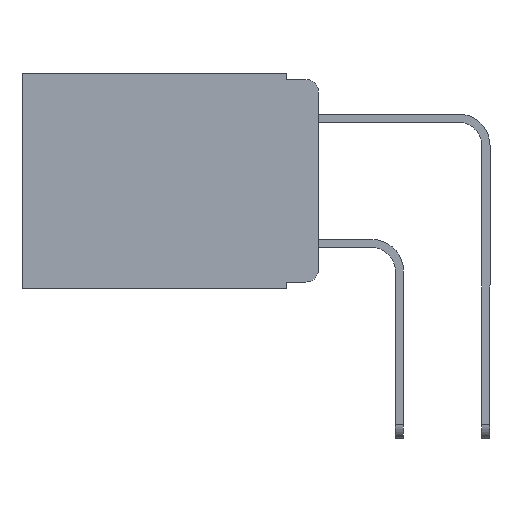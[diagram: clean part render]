
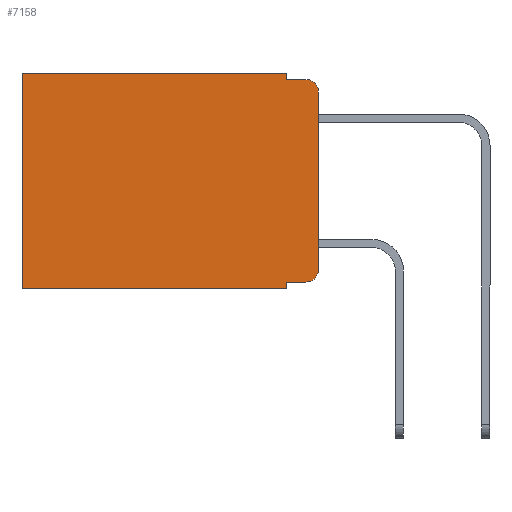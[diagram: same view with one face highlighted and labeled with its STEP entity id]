
A CAD part, left-side view. The second image highlights one B-rep face of the part: STEP entity #7158.
In plain terms, the highlighted planar face has unit normal (-1, 0, 0).
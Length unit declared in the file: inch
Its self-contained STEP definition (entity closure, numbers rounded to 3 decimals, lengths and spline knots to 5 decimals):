
#223 = ORIENTED_EDGE ( 'NONE', *, *, #5696, .T. ) ;
#335 = VERTEX_POINT ( 'NONE', #11684 ) ;
#1074 = VERTEX_POINT ( 'NONE', #4058 ) ;
#1845 = VERTEX_POINT ( 'NONE', #11970 ) ;
#2031 = CARTESIAN_POINT ( 'NONE',  ( 0.298, 0.051, -0.01 ) ) ;
#2078 = LINE ( 'NONE', #12561, #13362 ) ;
#2335 = CARTESIAN_POINT ( 'NONE',  ( 0.298, 0.051, 0. ) ) ;
#2446 = VECTOR ( 'NONE', #4903, 39.37008 ) ;
#2692 = DIRECTION ( 'NONE',  ( 0., 1., 0. ) ) ;
#2840 = LINE ( 'NONE', #9837, #10707 ) ;
#3233 = LINE ( 'NONE', #10443, #6314 ) ;
#3325 = PLANE ( 'NONE',  #10552 ) ;
#3360 = EDGE_CURVE ( 'NONE', #9661, #1074, #3486, .T. ) ;
#3486 = CIRCLE ( 'NONE', #14218, 0.02 ) ;
#3737 = CARTESIAN_POINT ( 'NONE',  ( 0.298, 0.051, -0.01 ) ) ;
#4058 = CARTESIAN_POINT ( 'NONE',  ( 0.298, 0., -0.313 ) ) ;
#4178 = EDGE_CURVE ( 'NONE', #1845, #9661, #5312, .T. ) ;
#4342 = DIRECTION ( 'NONE',  ( 0., 1., 0. ) ) ;
#4356 = VERTEX_POINT ( 'NONE', #3737 ) ;
#4550 = DIRECTION ( 'NONE',  ( 1., 0., 0. ) ) ;
#4607 = VERTEX_POINT ( 'NONE', #6567 ) ;
#4618 = CARTESIAN_POINT ( 'NONE',  ( 0.298, 0.473, 0. ) ) ;
#4702 = VECTOR ( 'NONE', #11023, 39.37008 ) ;
#4903 = DIRECTION ( 'NONE',  ( 0., 0., -1. ) ) ;
#4949 = VECTOR ( 'NONE', #11162, 39.37008 ) ;
#4968 = EDGE_CURVE ( 'NONE', #1845, #9438, #3233, .T. ) ;
#4982 = ORIENTED_EDGE ( 'NONE', *, *, #7124, .F. ) ;
#5066 = EDGE_CURVE ( 'NONE', #7900, #9487, #2078, .T. ) ;
#5312 = LINE ( 'NONE', #10072, #4949 ) ;
#5460 = CARTESIAN_POINT ( 'NONE',  ( 0.298, 0.02, -0.313 ) ) ;
#5696 = EDGE_CURVE ( 'NONE', #9487, #12836, #7772, .T. ) ;
#5735 = DIRECTION ( 'NONE',  ( -1., 0., 0. ) ) ;
#5866 = CARTESIAN_POINT ( 'NONE',  ( 0.298, 0.051, 0. ) ) ;
#5968 = LINE ( 'NONE', #10895, #12598 ) ;
#6314 = VECTOR ( 'NONE', #13435, 39.37008 ) ;
#6437 = EDGE_CURVE ( 'NONE', #7900, #4356, #7913, .T. ) ;
#6533 = ORIENTED_EDGE ( 'NONE', *, *, #6437, .F. ) ;
#6555 = DIRECTION ( 'NONE',  ( 0., 0., -1. ) ) ;
#6567 = CARTESIAN_POINT ( 'NONE',  ( 0.298, 0.02, -0.01 ) ) ;
#7124 = EDGE_CURVE ( 'NONE', #4356, #4607, #7585, .T. ) ;
#7158 = ADVANCED_FACE ( 'NONE', ( #7235 ), #3325, .F. ) ;
#7235 = FACE_OUTER_BOUND ( 'NONE', #9137, .T. ) ;
#7581 = VECTOR ( 'NONE', #14245, 39.37008 ) ;
#7585 = LINE ( 'NONE', #2031, #4702 ) ;
#7772 = LINE ( 'NONE', #10321, #2446 ) ;
#7847 = EDGE_CURVE ( 'NONE', #335, #4607, #8940, .T. ) ;
#7900 = VERTEX_POINT ( 'NONE', #2335 ) ;
#7913 = LINE ( 'NONE', #5866, #7581 ) ;
#8059 = CARTESIAN_POINT ( 'NONE',  ( 0.298, 0.02, -0.333 ) ) ;
#8377 = ORIENTED_EDGE ( 'NONE', *, *, #12076, .F. ) ;
#8737 = ORIENTED_EDGE ( 'NONE', *, *, #12150, .F. ) ;
#8831 = CARTESIAN_POINT ( 'NONE',  ( 0.298, 0.473, -0.343 ) ) ;
#8940 = CIRCLE ( 'NONE', #10730, 0.02 ) ;
#9137 = EDGE_LOOP ( 'NONE', ( #8737, #13190, #4982, #6533, #12044, #223, #8377, #13023, #14110, #10239 ) ) ;
#9438 = VERTEX_POINT ( 'NONE', #12053 ) ;
#9487 = VERTEX_POINT ( 'NONE', #4618 ) ;
#9661 = VERTEX_POINT ( 'NONE', #8059 ) ;
#9837 = CARTESIAN_POINT ( 'NONE',  ( 0.298, 0., 0. ) ) ;
#9883 = DIRECTION ( 'NONE',  ( 0., 0., -1. ) ) ;
#10072 = CARTESIAN_POINT ( 'NONE',  ( 0.298, 0.051, -0.333 ) ) ;
#10239 = ORIENTED_EDGE ( 'NONE', *, *, #3360, .T. ) ;
#10321 = CARTESIAN_POINT ( 'NONE',  ( 0.298, 0.473, 0. ) ) ;
#10443 = CARTESIAN_POINT ( 'NONE',  ( 0.298, 0.051, 0. ) ) ;
#10552 = AXIS2_PLACEMENT_3D ( 'NONE', #11075, #4550, #12079 ) ;
#10707 = VECTOR ( 'NONE', #9883, 39.37008 ) ;
#10730 = AXIS2_PLACEMENT_3D ( 'NONE', #12146, #5735, #13131 ) ;
#10895 = CARTESIAN_POINT ( 'NONE',  ( 0.298, 0., -0.343 ) ) ;
#11023 = DIRECTION ( 'NONE',  ( 0., -1., 0. ) ) ;
#11075 = CARTESIAN_POINT ( 'NONE',  ( 0.298, 0., 0. ) ) ;
#11162 = DIRECTION ( 'NONE',  ( 0., -1., 0. ) ) ;
#11684 = CARTESIAN_POINT ( 'NONE',  ( 0.298, 0., -0.03 ) ) ;
#11970 = CARTESIAN_POINT ( 'NONE',  ( 0.298, 0.051, -0.333 ) ) ;
#12044 = ORIENTED_EDGE ( 'NONE', *, *, #5066, .T. ) ;
#12053 = CARTESIAN_POINT ( 'NONE',  ( 0.298, 0.051, -0.343 ) ) ;
#12076 = EDGE_CURVE ( 'NONE', #9438, #12836, #5968, .T. ) ;
#12079 = DIRECTION ( 'NONE',  ( 0., 0., -1. ) ) ;
#12146 = CARTESIAN_POINT ( 'NONE',  ( 0.298, 0.02, -0.03 ) ) ;
#12150 = EDGE_CURVE ( 'NONE', #335, #1074, #2840, .T. ) ;
#12561 = CARTESIAN_POINT ( 'NONE',  ( 0.298, 0., 0. ) ) ;
#12598 = VECTOR ( 'NONE', #4342, 39.37008 ) ;
#12836 = VERTEX_POINT ( 'NONE', #8831 ) ;
#12869 = DIRECTION ( 'NONE',  ( -1., 0., 0. ) ) ;
#13023 = ORIENTED_EDGE ( 'NONE', *, *, #4968, .F. ) ;
#13131 = DIRECTION ( 'NONE',  ( 0., 0., -1. ) ) ;
#13190 = ORIENTED_EDGE ( 'NONE', *, *, #7847, .T. ) ;
#13362 = VECTOR ( 'NONE', #2692, 39.37008 ) ;
#13435 = DIRECTION ( 'NONE',  ( 0., 0., -1. ) ) ;
#14110 = ORIENTED_EDGE ( 'NONE', *, *, #4178, .T. ) ;
#14218 = AXIS2_PLACEMENT_3D ( 'NONE', #5460, #12869, #6555 ) ;
#14245 = DIRECTION ( 'NONE',  ( 0., 0., -1. ) ) ;
